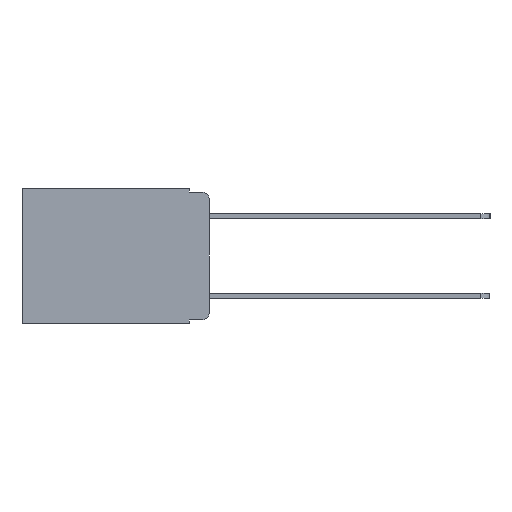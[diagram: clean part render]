
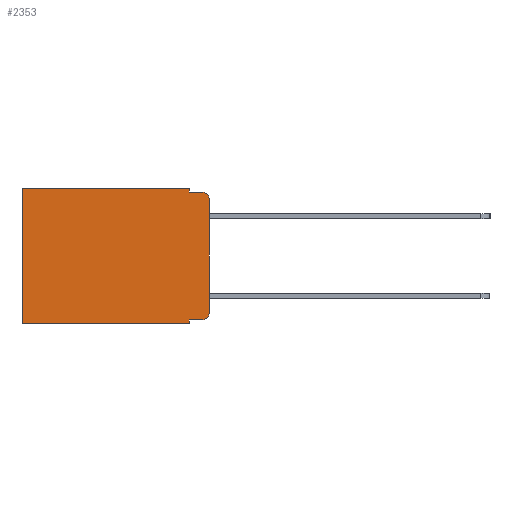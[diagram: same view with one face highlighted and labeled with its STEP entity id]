
A CAD part, left-side view. The second image highlights one B-rep face of the part: STEP entity #2353.
In plain terms, the highlighted planar face has unit normal (-1, 0, 0).
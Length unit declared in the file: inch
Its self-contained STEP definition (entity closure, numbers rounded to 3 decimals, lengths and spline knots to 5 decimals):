
#247 = VECTOR ( 'NONE', #2727, 39.37008 ) ;
#323 = DIRECTION ( 'NONE',  ( 0., 0., -1. ) ) ;
#416 = EDGE_CURVE ( 'NONE', #8769, #8786, #9483, .T. ) ;
#454 = VECTOR ( 'NONE', #4193, 39.37008 ) ;
#472 = VERTEX_POINT ( 'NONE', #10508 ) ;
#477 = LINE ( 'NONE', #6934, #4541 ) ;
#923 = LINE ( 'NONE', #5479, #454 ) ;
#1156 = CARTESIAN_POINT ( 'NONE',  ( 0.298, 0.051, -0.01 ) ) ;
#1235 = DIRECTION ( 'NONE',  ( 0., 0., -1. ) ) ;
#1479 = CARTESIAN_POINT ( 'NONE',  ( 0.298, 0.051, -0.343 ) ) ;
#1584 = CIRCLE ( 'NONE', #15141, 0.02 ) ;
#2353 = ADVANCED_FACE ( 'NONE', ( #15500 ), #3682, .F. ) ;
#2727 = DIRECTION ( 'NONE',  ( 0., -1., 0. ) ) ;
#3031 = EDGE_CURVE ( 'NONE', #14230, #15051, #8225, .T. ) ;
#3048 = CARTESIAN_POINT ( 'NONE',  ( 0.298, 0.02, -0.03 ) ) ;
#3146 = CARTESIAN_POINT ( 'NONE',  ( 0.298, 0., 0. ) ) ;
#3226 = DIRECTION ( 'NONE',  ( 0., 0., -1. ) ) ;
#3332 = VECTOR ( 'NONE', #12111, 39.37008 ) ;
#3682 = PLANE ( 'NONE',  #5818 ) ;
#3945 = LINE ( 'NONE', #7707, #247 ) ;
#3989 = LINE ( 'NONE', #6508, #7280 ) ;
#4120 = CARTESIAN_POINT ( 'NONE',  ( 0.298, 0.051, 0. ) ) ;
#4193 = DIRECTION ( 'NONE',  ( 0., 1., 0. ) ) ;
#4346 = DIRECTION ( 'NONE',  ( 0., 0., -1. ) ) ;
#4458 = VERTEX_POINT ( 'NONE', #13335 ) ;
#4541 = VECTOR ( 'NONE', #13996, 39.37008 ) ;
#4762 = CIRCLE ( 'NONE', #12638, 0.02 ) ;
#5479 = CARTESIAN_POINT ( 'NONE',  ( 0.298, 0., -0.343 ) ) ;
#5487 = CARTESIAN_POINT ( 'NONE',  ( 0.298, 0., -0.313 ) ) ;
#5528 = CARTESIAN_POINT ( 'NONE',  ( 0.298, 0.02, -0.313 ) ) ;
#5641 = CARTESIAN_POINT ( 'NONE',  ( 0.298, 0.051, 0. ) ) ;
#5785 = ORIENTED_EDGE ( 'NONE', *, *, #416, .T. ) ;
#5818 = AXIS2_PLACEMENT_3D ( 'NONE', #5834, #13667, #323 ) ;
#5834 = CARTESIAN_POINT ( 'NONE',  ( 0.298, 0., 0. ) ) ;
#5913 = EDGE_CURVE ( 'NONE', #13442, #11656, #1584, .T. ) ;
#6382 = VERTEX_POINT ( 'NONE', #1156 ) ;
#6508 = CARTESIAN_POINT ( 'NONE',  ( 0.298, 0.473, 0. ) ) ;
#6765 = DIRECTION ( 'NONE',  ( 0., 0., -1. ) ) ;
#6882 = VECTOR ( 'NONE', #12884, 39.37008 ) ;
#6934 = CARTESIAN_POINT ( 'NONE',  ( 0.298, 0.051, -0.333 ) ) ;
#7280 = VECTOR ( 'NONE', #14673, 39.37008 ) ;
#7707 = CARTESIAN_POINT ( 'NONE',  ( 0.298, 0.051, -0.01 ) ) ;
#8022 = ORIENTED_EDGE ( 'NONE', *, *, #3031, .F. ) ;
#8091 = EDGE_CURVE ( 'NONE', #8841, #11656, #15792, .T. ) ;
#8201 = ORIENTED_EDGE ( 'NONE', *, *, #8091, .F. ) ;
#8225 = LINE ( 'NONE', #4120, #12725 ) ;
#8578 = ORIENTED_EDGE ( 'NONE', *, *, #14206, .F. ) ;
#8679 = EDGE_CURVE ( 'NONE', #15051, #4458, #923, .T. ) ;
#8769 = VERTEX_POINT ( 'NONE', #5641 ) ;
#8786 = VERTEX_POINT ( 'NONE', #12863 ) ;
#8841 = VERTEX_POINT ( 'NONE', #10551 ) ;
#8944 = ORIENTED_EDGE ( 'NONE', *, *, #12231, .F. ) ;
#9483 = LINE ( 'NONE', #12299, #3332 ) ;
#9744 = LINE ( 'NONE', #11768, #12913 ) ;
#9885 = CARTESIAN_POINT ( 'NONE',  ( 0.298, 0.02, -0.333 ) ) ;
#10508 = CARTESIAN_POINT ( 'NONE',  ( 0.298, 0.02, -0.01 ) ) ;
#10551 = CARTESIAN_POINT ( 'NONE',  ( 0.298, 0., -0.03 ) ) ;
#11608 = DIRECTION ( 'NONE',  ( -1., 0., 0. ) ) ;
#11656 = VERTEX_POINT ( 'NONE', #5487 ) ;
#11768 = CARTESIAN_POINT ( 'NONE',  ( 0.298, 0.051, 0. ) ) ;
#11967 = ORIENTED_EDGE ( 'NONE', *, *, #5913, .T. ) ;
#12111 = DIRECTION ( 'NONE',  ( 0., 1., 0. ) ) ;
#12231 = EDGE_CURVE ( 'NONE', #8769, #6382, #9744, .T. ) ;
#12299 = CARTESIAN_POINT ( 'NONE',  ( 0.298, 0., 0. ) ) ;
#12638 = AXIS2_PLACEMENT_3D ( 'NONE', #3048, #11608, #4346 ) ;
#12725 = VECTOR ( 'NONE', #1235, 39.37008 ) ;
#12863 = CARTESIAN_POINT ( 'NONE',  ( 0.298, 0.473, 0. ) ) ;
#12884 = DIRECTION ( 'NONE',  ( 0., 0., -1. ) ) ;
#12913 = VECTOR ( 'NONE', #3226, 39.37008 ) ;
#13011 = EDGE_CURVE ( 'NONE', #8786, #4458, #3989, .T. ) ;
#13335 = CARTESIAN_POINT ( 'NONE',  ( 0.298, 0.473, -0.343 ) ) ;
#13442 = VERTEX_POINT ( 'NONE', #9885 ) ;
#13667 = DIRECTION ( 'NONE',  ( 1., 0., 0. ) ) ;
#13738 = EDGE_CURVE ( 'NONE', #8841, #472, #4762, .T. ) ;
#13796 = EDGE_LOOP ( 'NONE', ( #8201, #14095, #8578, #8944, #5785, #15461, #14260, #8022, #14591, #11967 ) ) ;
#13830 = DIRECTION ( 'NONE',  ( -1., 0., 0. ) ) ;
#13996 = DIRECTION ( 'NONE',  ( 0., -1., 0. ) ) ;
#14095 = ORIENTED_EDGE ( 'NONE', *, *, #13738, .T. ) ;
#14206 = EDGE_CURVE ( 'NONE', #6382, #472, #3945, .T. ) ;
#14230 = VERTEX_POINT ( 'NONE', #14736 ) ;
#14260 = ORIENTED_EDGE ( 'NONE', *, *, #8679, .F. ) ;
#14466 = EDGE_CURVE ( 'NONE', #14230, #13442, #477, .T. ) ;
#14591 = ORIENTED_EDGE ( 'NONE', *, *, #14466, .T. ) ;
#14673 = DIRECTION ( 'NONE',  ( 0., 0., -1. ) ) ;
#14736 = CARTESIAN_POINT ( 'NONE',  ( 0.298, 0.051, -0.333 ) ) ;
#15051 = VERTEX_POINT ( 'NONE', #1479 ) ;
#15141 = AXIS2_PLACEMENT_3D ( 'NONE', #5528, #13830, #6765 ) ;
#15461 = ORIENTED_EDGE ( 'NONE', *, *, #13011, .T. ) ;
#15500 = FACE_OUTER_BOUND ( 'NONE', #13796, .T. ) ;
#15792 = LINE ( 'NONE', #3146, #6882 ) ;
